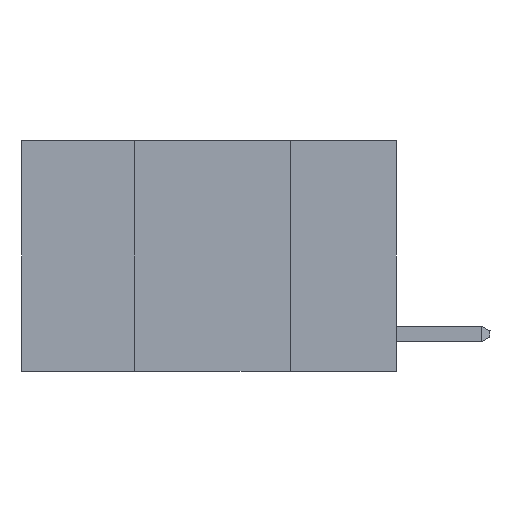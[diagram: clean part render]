
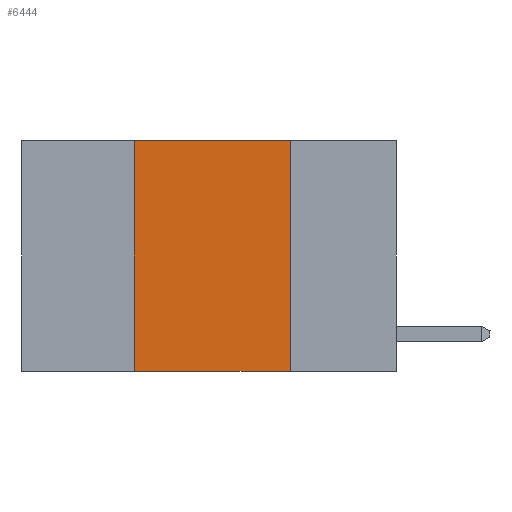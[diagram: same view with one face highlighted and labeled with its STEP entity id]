
A CAD part, left-side view. The second image highlights one B-rep face of the part: STEP entity #6444.
In plain terms, the highlighted planar face has unit normal (-1, 0, 0).
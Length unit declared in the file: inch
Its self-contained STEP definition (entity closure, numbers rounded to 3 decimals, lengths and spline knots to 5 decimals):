
#224 = LINE ( 'NONE', #29470, #13124 ) ;
#753 = ORIENTED_EDGE ( 'NONE', *, *, #8662, .F. ) ;
#2306 = PLANE ( 'NONE',  #24106 ) ;
#2353 = VERTEX_POINT ( 'NONE', #27210 ) ;
#3181 = VECTOR ( 'NONE', #18041, 39.37008 ) ;
#3270 = CARTESIAN_POINT ( 'NONE',  ( 0., 0.42, 0. ) ) ;
#4194 = CARTESIAN_POINT ( 'NONE',  ( 0., 0.6, 0. ) ) ;
#6436 = CARTESIAN_POINT ( 'NONE',  ( 0., 0.17, -0.37 ) ) ;
#6444 = ADVANCED_FACE ( 'NONE', ( #24818 ), #2306, .F. ) ;
#8631 = LINE ( 'NONE', #13144, #28346 ) ;
#8662 = EDGE_CURVE ( 'NONE', #27929, #13323, #224, .T. ) ;
#9626 = ORIENTED_EDGE ( 'NONE', *, *, #27887, .T. ) ;
#10822 = ORIENTED_EDGE ( 'NONE', *, *, #21339, .F. ) ;
#11268 = CARTESIAN_POINT ( 'NONE',  ( 0., 0.42, -0.37 ) ) ;
#13124 = VECTOR ( 'NONE', #27355, 39.37008 ) ;
#13144 = CARTESIAN_POINT ( 'NONE',  ( 0., 0.17, 0. ) ) ;
#13323 = VERTEX_POINT ( 'NONE', #3270 ) ;
#13697 = DIRECTION ( 'NONE',  ( 1., 0., 0. ) ) ;
#16152 = VECTOR ( 'NONE', #21751, 39.37008 ) ;
#17809 = DIRECTION ( 'NONE',  ( 0., 0., -1. ) ) ;
#18041 = DIRECTION ( 'NONE',  ( 0., -1., 0. ) ) ;
#18626 = CARTESIAN_POINT ( 'NONE',  ( 0., 0.6, -0.37 ) ) ;
#19972 = EDGE_LOOP ( 'NONE', ( #10822, #27882, #753, #9626 ) ) ;
#20171 = DIRECTION ( 'NONE',  ( 0., 0., -1. ) ) ;
#21339 = EDGE_CURVE ( 'NONE', #2353, #25149, #8631, .T. ) ;
#21751 = DIRECTION ( 'NONE',  ( 0., -1., 0. ) ) ;
#23100 = LINE ( 'NONE', #18626, #3181 ) ;
#24106 = AXIS2_PLACEMENT_3D ( 'NONE', #27476, #13697, #20171 ) ;
#24739 = LINE ( 'NONE', #4194, #16152 ) ;
#24818 = FACE_OUTER_BOUND ( 'NONE', #19972, .T. ) ;
#25149 = VERTEX_POINT ( 'NONE', #6436 ) ;
#27210 = CARTESIAN_POINT ( 'NONE',  ( 0., 0.17, 0. ) ) ;
#27355 = DIRECTION ( 'NONE',  ( 0., 0., 1. ) ) ;
#27476 = CARTESIAN_POINT ( 'NONE',  ( 0., 0.6, 0. ) ) ;
#27882 = ORIENTED_EDGE ( 'NONE', *, *, #28240, .F. ) ;
#27887 = EDGE_CURVE ( 'NONE', #27929, #25149, #23100, .T. ) ;
#27929 = VERTEX_POINT ( 'NONE', #11268 ) ;
#28240 = EDGE_CURVE ( 'NONE', #13323, #2353, #24739, .T. ) ;
#28346 = VECTOR ( 'NONE', #17809, 39.37008 ) ;
#29470 = CARTESIAN_POINT ( 'NONE',  ( 0., 0.42, 0. ) ) ;
